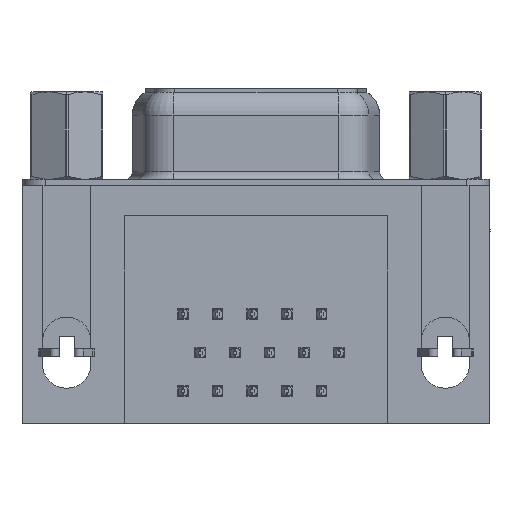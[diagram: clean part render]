
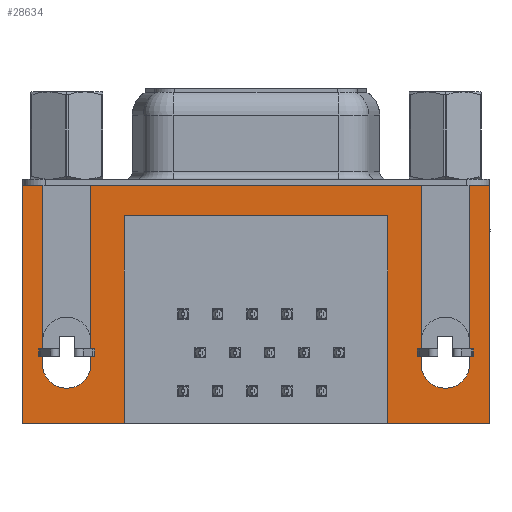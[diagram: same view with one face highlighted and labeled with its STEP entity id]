
A CAD part, front view. The second image highlights one B-rep face of the part: STEP entity #28634.
In plain terms, the highlighted planar face has unit normal (0, -1, 0).
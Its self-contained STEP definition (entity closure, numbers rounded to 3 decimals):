
#355 = VECTOR ( 'NONE', #13934, 1000. ) ;
#674 = DIRECTION ( 'NONE',  ( 0., -1., 0. ) ) ;
#768 = CARTESIAN_POINT ( 'NONE',  ( 23.39, -6.275, 0. ) ) ;
#915 = EDGE_CURVE ( 'NONE', #25374, #15934, #16794, .T. ) ;
#1068 = CARTESIAN_POINT ( 'NONE',  ( 0., -6.275, -11.78 ) ) ;
#1212 = LINE ( 'NONE', #42275, #35908 ) ;
#1403 = DIRECTION ( 'NONE',  ( 0., 0., 1. ) ) ;
#1622 = VERTEX_POINT ( 'NONE', #22244 ) ;
#1857 = ORIENTED_EDGE ( 'NONE', *, *, #915, .F. ) ;
#2195 = DIRECTION ( 'NONE',  ( 1., 0., 0. ) ) ;
#2200 = DIRECTION ( 'NONE',  ( 0., 0., -1. ) ) ;
#2334 = CARTESIAN_POINT ( 'NONE',  ( 1.6, -6.275, -11.78 ) ) ;
#2504 = DIRECTION ( 'NONE',  ( 0., -1., 0. ) ) ;
#3329 = LINE ( 'NONE', #7789, #13121 ) ;
#3395 = CARTESIAN_POINT ( 'NONE',  ( -2.91, -6.275, 0. ) ) ;
#4510 = VECTOR ( 'NONE', #13181, 1000. ) ;
#4773 = CARTESIAN_POINT ( 'NONE',  ( -2.91, -6.275, -2.5 ) ) ;
#5076 = VECTOR ( 'NONE', #18215, 1000. ) ;
#5457 = EDGE_CURVE ( 'NONE', #27652, #28214, #11502, .T. ) ;
#5733 = ORIENTED_EDGE ( 'NONE', *, *, #34388, .F. ) ;
#5781 = ORIENTED_EDGE ( 'NONE', *, *, #26558, .T. ) ;
#6341 = VECTOR ( 'NONE', #12902, 1000. ) ;
#6620 = CARTESIAN_POINT ( 'NONE',  ( 23.39, -6.275, -11.78 ) ) ;
#6832 = FACE_OUTER_BOUND ( 'NONE', #38025, .T. ) ;
#6958 = CARTESIAN_POINT ( 'NONE',  ( 27.9, -6.275, -15.7 ) ) ;
#7144 = VERTEX_POINT ( 'NONE', #13361 ) ;
#7149 = CARTESIAN_POINT ( 'NONE',  ( 3.79, -6.275, -2. ) ) ;
#7449 = DIRECTION ( 'NONE',  ( 0., 0., -1. ) ) ;
#7615 = ORIENTED_EDGE ( 'NONE', *, *, #22199, .F. ) ;
#7789 = CARTESIAN_POINT ( 'NONE',  ( 27.9, -6.275, -2.5 ) ) ;
#7842 = LINE ( 'NONE', #37809, #41389 ) ;
#7959 = CARTESIAN_POINT ( 'NONE',  ( -1.6, -6.275, 0. ) ) ;
#8235 = VERTEX_POINT ( 'NONE', #34158 ) ;
#8346 = LINE ( 'NONE', #9621, #6341 ) ;
#8414 = ORIENTED_EDGE ( 'NONE', *, *, #10046, .F. ) ;
#9197 = CIRCLE ( 'NONE', #33133, 1.6 ) ;
#9239 = VECTOR ( 'NONE', #31652, 1000. ) ;
#9307 = CARTESIAN_POINT ( 'NONE',  ( 3.79, -6.275, -2. ) ) ;
#9621 = CARTESIAN_POINT ( 'NONE',  ( 3.79, -6.275, -2. ) ) ;
#9948 = ORIENTED_EDGE ( 'NONE', *, *, #5457, .F. ) ;
#10046 = EDGE_CURVE ( 'NONE', #28214, #19630, #13825, .T. ) ;
#10289 = DIRECTION ( 'NONE',  ( -1., 0., 0. ) ) ;
#11502 = CIRCLE ( 'NONE', #39911, 1.6 ) ;
#11880 = CARTESIAN_POINT ( 'NONE',  ( 1.6, -6.275, 0. ) ) ;
#12902 = DIRECTION ( 'NONE',  ( -1., 0., 0. ) ) ;
#13121 = VECTOR ( 'NONE', #30500, 1000. ) ;
#13181 = DIRECTION ( 'NONE',  ( 1., 0., 0. ) ) ;
#13361 = CARTESIAN_POINT ( 'NONE',  ( 27.9, -6.275, -15.7 ) ) ;
#13825 = LINE ( 'NONE', #11880, #5076 ) ;
#13916 = LINE ( 'NONE', #38371, #38755 ) ;
#13934 = DIRECTION ( 'NONE',  ( 0., 0., 1. ) ) ;
#14262 = VECTOR ( 'NONE', #26178, 1000. ) ;
#14450 = EDGE_CURVE ( 'NONE', #1622, #18546, #30449, .T. ) ;
#14456 = EDGE_CURVE ( 'NONE', #30332, #31195, #39125, .T. ) ;
#14987 = EDGE_CURVE ( 'NONE', #7144, #25374, #17249, .T. ) ;
#15934 = VERTEX_POINT ( 'NONE', #18048 ) ;
#16473 = DIRECTION ( 'NONE',  ( 0., 0., 1. ) ) ;
#16594 = EDGE_CURVE ( 'NONE', #29589, #30332, #1212, .T. ) ;
#16794 = LINE ( 'NONE', #17535, #355 ) ;
#16855 = CARTESIAN_POINT ( 'NONE',  ( 27.9, -6.275, 0. ) ) ;
#17249 = LINE ( 'NONE', #6958, #33532 ) ;
#17289 = LINE ( 'NONE', #9307, #23903 ) ;
#17535 = CARTESIAN_POINT ( 'NONE',  ( 21.2, -6.275, -2. ) ) ;
#17815 = LINE ( 'NONE', #28377, #9239 ) ;
#18048 = CARTESIAN_POINT ( 'NONE',  ( 21.2, -6.275, -2. ) ) ;
#18161 = CARTESIAN_POINT ( 'NONE',  ( -2.91, -6.275, -2.5 ) ) ;
#18215 = DIRECTION ( 'NONE',  ( 0., 0., 1. ) ) ;
#18418 = CARTESIAN_POINT ( 'NONE',  ( 26.59, -6.275, 0. ) ) ;
#18546 = VERTEX_POINT ( 'NONE', #7959 ) ;
#18801 = CARTESIAN_POINT ( 'NONE',  ( 1.6, -6.275, 0. ) ) ;
#18929 = DIRECTION ( 'NONE',  ( -1., 0., 0. ) ) ;
#18969 = VERTEX_POINT ( 'NONE', #19462 ) ;
#19462 = CARTESIAN_POINT ( 'NONE',  ( -2.91, -6.275, -15.7 ) ) ;
#19570 = EDGE_CURVE ( 'NONE', #18546, #27652, #7842, .T. ) ;
#19630 = VERTEX_POINT ( 'NONE', #18801 ) ;
#19645 = CARTESIAN_POINT ( 'NONE',  ( -2.91, -6.275, 0. ) ) ;
#20303 = CARTESIAN_POINT ( 'NONE',  ( -1.6, -6.275, -11.78 ) ) ;
#20678 = VERTEX_POINT ( 'NONE', #33665 ) ;
#20917 = ORIENTED_EDGE ( 'NONE', *, *, #16594, .F. ) ;
#20995 = VERTEX_POINT ( 'NONE', #6620 ) ;
#21414 = VERTEX_POINT ( 'NONE', #7149 ) ;
#21448 = DIRECTION ( 'NONE',  ( 0., 0., -1. ) ) ;
#21889 = VECTOR ( 'NONE', #7449, 1000. ) ;
#22087 = CARTESIAN_POINT ( 'NONE',  ( 24.99, -6.275, -11.78 ) ) ;
#22199 = EDGE_CURVE ( 'NONE', #20678, #20995, #38744, .T. ) ;
#22244 = CARTESIAN_POINT ( 'NONE',  ( -2.91, -6.275, 0. ) ) ;
#22983 = ORIENTED_EDGE ( 'NONE', *, *, #14450, .F. ) ;
#23849 = EDGE_CURVE ( 'NONE', #18969, #1622, #39162, .T. ) ;
#23903 = VECTOR ( 'NONE', #28724, 1000. ) ;
#24720 = ORIENTED_EDGE ( 'NONE', *, *, #33738, .F. ) ;
#24904 = VECTOR ( 'NONE', #1403, 1000. ) ;
#25341 = DIRECTION ( 'NONE',  ( -1., 0., 0. ) ) ;
#25374 = VERTEX_POINT ( 'NONE', #38986 ) ;
#26178 = DIRECTION ( 'NONE',  ( 1., 0., 0. ) ) ;
#26558 = EDGE_CURVE ( 'NONE', #7144, #31195, #3329, .T. ) ;
#27652 = VERTEX_POINT ( 'NONE', #20303 ) ;
#28214 = VERTEX_POINT ( 'NONE', #2334 ) ;
#28217 = ORIENTED_EDGE ( 'NONE', *, *, #34774, .F. ) ;
#28293 = EDGE_CURVE ( 'NONE', #15934, #21414, #8346, .T. ) ;
#28377 = CARTESIAN_POINT ( 'NONE',  ( -2.91, -6.275, 0. ) ) ;
#28634 = ADVANCED_FACE ( 'NONE', ( #6832 ), #34252, .T. ) ;
#28724 = DIRECTION ( 'NONE',  ( 0., 0., -1. ) ) ;
#29589 = VERTEX_POINT ( 'NONE', #40369 ) ;
#30332 = VERTEX_POINT ( 'NONE', #18418 ) ;
#30449 = LINE ( 'NONE', #3395, #14262 ) ;
#30500 = DIRECTION ( 'NONE',  ( 0., 0., 1. ) ) ;
#31195 = VERTEX_POINT ( 'NONE', #16855 ) ;
#31652 = DIRECTION ( 'NONE',  ( 1., 0., 0. ) ) ;
#32655 = ORIENTED_EDGE ( 'NONE', *, *, #23849, .F. ) ;
#33114 = ORIENTED_EDGE ( 'NONE', *, *, #14456, .F. ) ;
#33133 = AXIS2_PLACEMENT_3D ( 'NONE', #22087, #2504, #25341 ) ;
#33347 = ORIENTED_EDGE ( 'NONE', *, *, #41247, .F. ) ;
#33532 = VECTOR ( 'NONE', #10289, 1000. ) ;
#33665 = CARTESIAN_POINT ( 'NONE',  ( 23.39, -6.275, 0. ) ) ;
#33738 = EDGE_CURVE ( 'NONE', #19630, #20678, #17815, .T. ) ;
#34158 = CARTESIAN_POINT ( 'NONE',  ( 3.79, -6.275, -15.7 ) ) ;
#34252 = PLANE ( 'NONE',  #37512 ) ;
#34388 = EDGE_CURVE ( 'NONE', #20995, #29589, #9197, .T. ) ;
#34774 = EDGE_CURVE ( 'NONE', #21414, #8235, #17289, .T. ) ;
#35908 = VECTOR ( 'NONE', #16473, 1000. ) ;
#37512 = AXIS2_PLACEMENT_3D ( 'NONE', #18161, #40912, #21448 ) ;
#37640 = ORIENTED_EDGE ( 'NONE', *, *, #14987, .F. ) ;
#37809 = CARTESIAN_POINT ( 'NONE',  ( -1.6, -6.275, 0. ) ) ;
#38025 = EDGE_LOOP ( 'NONE', ( #20917, #5733, #7615, #24720, #8414, #9948, #42244, #22983, #32655, #33347, #28217, #38519, #1857, #37640, #5781, #33114 ) ) ;
#38371 = CARTESIAN_POINT ( 'NONE',  ( 27.9, -6.275, -15.7 ) ) ;
#38519 = ORIENTED_EDGE ( 'NONE', *, *, #28293, .F. ) ;
#38744 = LINE ( 'NONE', #768, #21889 ) ;
#38755 = VECTOR ( 'NONE', #18929, 1000. ) ;
#38986 = CARTESIAN_POINT ( 'NONE',  ( 21.2, -6.275, -15.7 ) ) ;
#39125 = LINE ( 'NONE', #19645, #4510 ) ;
#39162 = LINE ( 'NONE', #4773, #24904 ) ;
#39911 = AXIS2_PLACEMENT_3D ( 'NONE', #1068, #674, #2195 ) ;
#40369 = CARTESIAN_POINT ( 'NONE',  ( 26.59, -6.275, -11.78 ) ) ;
#40912 = DIRECTION ( 'NONE',  ( 0., -1., 0. ) ) ;
#41247 = EDGE_CURVE ( 'NONE', #8235, #18969, #13916, .T. ) ;
#41389 = VECTOR ( 'NONE', #2200, 1000. ) ;
#42244 = ORIENTED_EDGE ( 'NONE', *, *, #19570, .F. ) ;
#42275 = CARTESIAN_POINT ( 'NONE',  ( 26.59, -6.275, 0. ) ) ;
